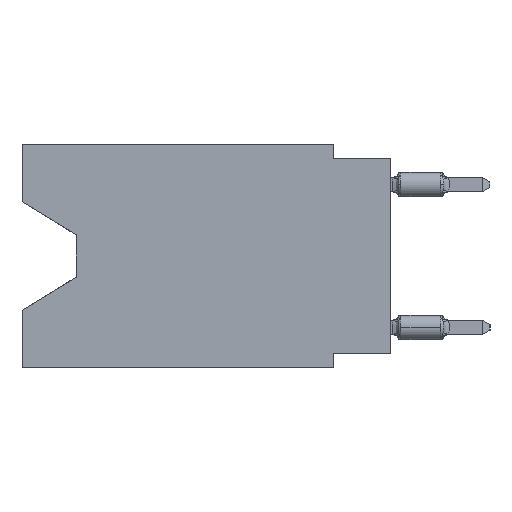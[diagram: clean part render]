
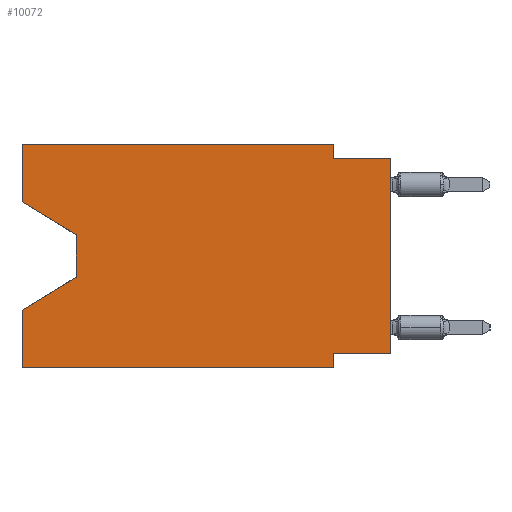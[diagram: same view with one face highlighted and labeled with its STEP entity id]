
A CAD part, left-side view. The second image highlights one B-rep face of the part: STEP entity #10072.
In plain terms, the highlighted planar face has unit normal (-1, 0, 0).
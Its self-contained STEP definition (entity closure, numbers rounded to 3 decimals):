
#50 = EDGE_CURVE ( 'NONE', #11829, #12048, #8824, .T. ) ;
#939 = EDGE_CURVE ( 'NONE', #5467, #2951, #25495, .T. ) ;
#1751 = ORIENTED_EDGE ( 'NONE', *, *, #25366, .F. ) ;
#2052 = ORIENTED_EDGE ( 'NONE', *, *, #30627, .F. ) ;
#2951 = VERTEX_POINT ( 'NONE', #18516 ) ;
#3074 = VECTOR ( 'NONE', #34275, 1000. ) ;
#3738 = ORIENTED_EDGE ( 'NONE', *, *, #939, .T. ) ;
#3812 = VECTOR ( 'NONE', #7223, 1000. ) ;
#5177 = VERTEX_POINT ( 'NONE', #30625 ) ;
#5362 = DIRECTION ( 'NONE',  ( 0., 0., -1. ) ) ;
#5467 = VERTEX_POINT ( 'NONE', #35162 ) ;
#6039 = CARTESIAN_POINT ( 'NONE',  ( 0., 16.383, 0. ) ) ;
#6376 = DIRECTION ( 'NONE',  ( 0., 0., -1. ) ) ;
#7047 = CARTESIAN_POINT ( 'NONE',  ( 0., 16.383, -2.546 ) ) ;
#7112 = EDGE_CURVE ( 'NONE', #12255, #8151, #11734, .T. ) ;
#7223 = DIRECTION ( 'NONE',  ( 0., -0.855, -0.519 ) ) ;
#8052 = PLANE ( 'NONE',  #21398 ) ;
#8151 = VERTEX_POINT ( 'NONE', #34000 ) ;
#8633 = DIRECTION ( 'NONE',  ( 0., -1., 0. ) ) ;
#8824 = LINE ( 'NONE', #6039, #14077 ) ;
#8870 = DIRECTION ( 'NONE',  ( 0., 0., -1. ) ) ;
#9052 = VECTOR ( 'NONE', #9745, 1000. ) ;
#9375 = VECTOR ( 'NONE', #23846, 1000. ) ;
#9573 = VECTOR ( 'NONE', #15627, 1000. ) ;
#9745 = DIRECTION ( 'NONE',  ( 0., 1., 0. ) ) ;
#10003 = CARTESIAN_POINT ( 'NONE',  ( 0., 13.97, -5.893 ) ) ;
#10072 = ADVANCED_FACE ( 'NONE', ( #10823 ), #8052, .F. ) ;
#10723 = LINE ( 'NONE', #22284, #16469 ) ;
#10823 = FACE_OUTER_BOUND ( 'NONE', #20728, .T. ) ;
#11391 = ORIENTED_EDGE ( 'NONE', *, *, #50, .F. ) ;
#11734 = LINE ( 'NONE', #28701, #19587 ) ;
#11829 = VERTEX_POINT ( 'NONE', #30171 ) ;
#11831 = LINE ( 'NONE', #17428, #16772 ) ;
#11862 = EDGE_CURVE ( 'NONE', #34080, #31000, #30347, .T. ) ;
#11935 = CARTESIAN_POINT ( 'NONE',  ( 0., 16.383, 0. ) ) ;
#12048 = VERTEX_POINT ( 'NONE', #17487 ) ;
#12125 = LINE ( 'NONE', #31884, #22810 ) ;
#12255 = VERTEX_POINT ( 'NONE', #10003 ) ;
#12512 = ORIENTED_EDGE ( 'NONE', *, *, #31552, .T. ) ;
#12532 = LINE ( 'NONE', #35269, #9052 ) ;
#13576 = EDGE_CURVE ( 'NONE', #13862, #2951, #11831, .T. ) ;
#13693 = EDGE_CURVE ( 'NONE', #26764, #13862, #12532, .T. ) ;
#13862 = VERTEX_POINT ( 'NONE', #22036 ) ;
#14077 = VECTOR ( 'NONE', #8633, 1000. ) ;
#14663 = DIRECTION ( 'NONE',  ( 0., -1., 0. ) ) ;
#14878 = DIRECTION ( 'NONE',  ( 0., 0.855, -0.519 ) ) ;
#15627 = DIRECTION ( 'NONE',  ( 0., -1., 0. ) ) ;
#15721 = DIRECTION ( 'NONE',  ( 0., 0., 1. ) ) ;
#16323 = DIRECTION ( 'NONE',  ( 0., 0., -1. ) ) ;
#16469 = VECTOR ( 'NONE', #16323, 1000. ) ;
#16772 = VECTOR ( 'NONE', #8870, 1000. ) ;
#16774 = EDGE_CURVE ( 'NONE', #5177, #12255, #25462, .T. ) ;
#17131 = EDGE_CURVE ( 'NONE', #26764, #31000, #28889, .T. ) ;
#17308 = ORIENTED_EDGE ( 'NONE', *, *, #13693, .F. ) ;
#17428 = CARTESIAN_POINT ( 'NONE',  ( 0., 2.54, -9.906 ) ) ;
#17487 = CARTESIAN_POINT ( 'NONE',  ( 0., 2.54, 0. ) ) ;
#18248 = CARTESIAN_POINT ( 'NONE',  ( 0., 2.54, -0.635 ) ) ;
#18516 = CARTESIAN_POINT ( 'NONE',  ( 0., 2.54, -9.906 ) ) ;
#19072 = ORIENTED_EDGE ( 'NONE', *, *, #11862, .F. ) ;
#19414 = CARTESIAN_POINT ( 'NONE',  ( 0., 16.383, 0. ) ) ;
#19587 = VECTOR ( 'NONE', #14878, 1000. ) ;
#20142 = CARTESIAN_POINT ( 'NONE',  ( 0., 0., 0. ) ) ;
#20728 = EDGE_LOOP ( 'NONE', ( #12512, #20852, #23896, #2052, #3738, #25931, #17308, #30045, #19072, #22059, #11391, #1751 ) ) ;
#20852 = ORIENTED_EDGE ( 'NONE', *, *, #16774, .T. ) ;
#21398 = AXIS2_PLACEMENT_3D ( 'NONE', #19414, #30774, #6376 ) ;
#22034 = CARTESIAN_POINT ( 'NONE',  ( 0., 16.383, -9.906 ) ) ;
#22036 = CARTESIAN_POINT ( 'NONE',  ( 0., 2.54, -9.271 ) ) ;
#22059 = ORIENTED_EDGE ( 'NONE', *, *, #28459, .F. ) ;
#22284 = CARTESIAN_POINT ( 'NONE',  ( 0., 2.54, 0. ) ) ;
#22802 = CARTESIAN_POINT ( 'NONE',  ( 0., 0., -0.635 ) ) ;
#22810 = VECTOR ( 'NONE', #15721, 1000. ) ;
#23846 = DIRECTION ( 'NONE',  ( 0., 0., 1. ) ) ;
#23896 = ORIENTED_EDGE ( 'NONE', *, *, #7112, .T. ) ;
#24403 = VECTOR ( 'NONE', #5362, 1000. ) ;
#25366 = EDGE_CURVE ( 'NONE', #29934, #11829, #35028, .T. ) ;
#25462 = LINE ( 'NONE', #33271, #24403 ) ;
#25495 = LINE ( 'NONE', #22034, #31894 ) ;
#25931 = ORIENTED_EDGE ( 'NONE', *, *, #13576, .F. ) ;
#26084 = CARTESIAN_POINT ( 'NONE',  ( 0., 16.383, -2.546 ) ) ;
#26764 = VERTEX_POINT ( 'NONE', #28628 ) ;
#28459 = EDGE_CURVE ( 'NONE', #12048, #34080, #10723, .T. ) ;
#28628 = CARTESIAN_POINT ( 'NONE',  ( 0., 0., -9.271 ) ) ;
#28701 = CARTESIAN_POINT ( 'NONE',  ( 0., 13.97, -5.893 ) ) ;
#28889 = LINE ( 'NONE', #20142, #3074 ) ;
#29934 = VERTEX_POINT ( 'NONE', #26084 ) ;
#30045 = ORIENTED_EDGE ( 'NONE', *, *, #17131, .T. ) ;
#30171 = CARTESIAN_POINT ( 'NONE',  ( 0., 16.383, 0. ) ) ;
#30347 = LINE ( 'NONE', #32591, #9573 ) ;
#30625 = CARTESIAN_POINT ( 'NONE',  ( 0., 13.97, -4.013 ) ) ;
#30627 = EDGE_CURVE ( 'NONE', #5467, #8151, #12125, .T. ) ;
#30774 = DIRECTION ( 'NONE',  ( 1., 0., 0. ) ) ;
#31000 = VERTEX_POINT ( 'NONE', #22802 ) ;
#31552 = EDGE_CURVE ( 'NONE', #29934, #5177, #33279, .T. ) ;
#31884 = CARTESIAN_POINT ( 'NONE',  ( 0., 16.383, 0. ) ) ;
#31894 = VECTOR ( 'NONE', #14663, 1000. ) ;
#32591 = CARTESIAN_POINT ( 'NONE',  ( 0., 0., -0.635 ) ) ;
#33271 = CARTESIAN_POINT ( 'NONE',  ( 0., 13.97, -4.013 ) ) ;
#33279 = LINE ( 'NONE', #7047, #3812 ) ;
#34000 = CARTESIAN_POINT ( 'NONE',  ( 0., 16.383, -7.36 ) ) ;
#34080 = VERTEX_POINT ( 'NONE', #18248 ) ;
#34275 = DIRECTION ( 'NONE',  ( 0., 0., 1. ) ) ;
#35028 = LINE ( 'NONE', #11935, #9375 ) ;
#35162 = CARTESIAN_POINT ( 'NONE',  ( 0., 16.383, -9.906 ) ) ;
#35269 = CARTESIAN_POINT ( 'NONE',  ( 0., 0., -9.271 ) ) ;
